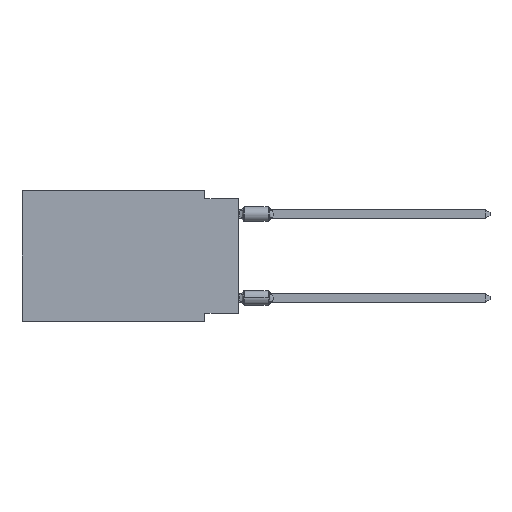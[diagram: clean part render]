
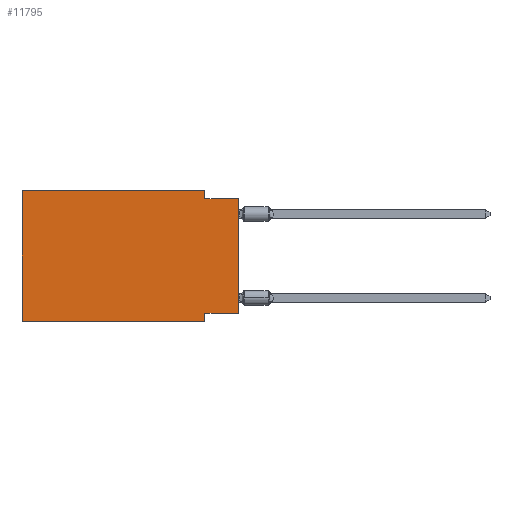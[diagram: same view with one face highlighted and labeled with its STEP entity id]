
A CAD part, left-side view. The second image highlights one B-rep face of the part: STEP entity #11795.
In plain terms, the highlighted planar face has unit normal (-1, 0, 0).
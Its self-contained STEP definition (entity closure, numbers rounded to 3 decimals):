
#19 = CARTESIAN_POINT ( 'NONE',  ( 0., 16.383, -9.906 ) ) ;
#109 = VECTOR ( 'NONE', #7532, 1000. ) ;
#499 = CARTESIAN_POINT ( 'NONE',  ( 0., 16.383, 0. ) ) ;
#580 = LINE ( 'NONE', #8457, #109 ) ;
#931 = EDGE_CURVE ( 'NONE', #2852, #11022, #6724, .T. ) ;
#1027 = DIRECTION ( 'NONE',  ( 0., -1., 0. ) ) ;
#1090 = LINE ( 'NONE', #4879, #1158 ) ;
#1113 = ORIENTED_EDGE ( 'NONE', *, *, #6436, .F. ) ;
#1158 = VECTOR ( 'NONE', #1027, 1000. ) ;
#1318 = ORIENTED_EDGE ( 'NONE', *, *, #931, .F. ) ;
#1481 = FACE_OUTER_BOUND ( 'NONE', #1704, .T. ) ;
#1704 = EDGE_LOOP ( 'NONE', ( #9704, #12590, #1318, #1113, #11437, #2610, #9833, #10017 ) ) ;
#1799 = DIRECTION ( 'NONE',  ( 0., 0., 1. ) ) ;
#1854 = LINE ( 'NONE', #12952, #9113 ) ;
#1952 = EDGE_CURVE ( 'NONE', #9389, #4710, #11287, .T. ) ;
#2149 = AXIS2_PLACEMENT_3D ( 'NONE', #499, #3488, #4475 ) ;
#2191 = LINE ( 'NONE', #7188, #9335 ) ;
#2273 = DIRECTION ( 'NONE',  ( 0., 0., 1. ) ) ;
#2501 = CARTESIAN_POINT ( 'NONE',  ( 0., 2.54, 0. ) ) ;
#2610 = ORIENTED_EDGE ( 'NONE', *, *, #7211, .T. ) ;
#2852 = VERTEX_POINT ( 'NONE', #6192 ) ;
#3065 = CARTESIAN_POINT ( 'NONE',  ( 0., 2.54, -0.635 ) ) ;
#3488 = DIRECTION ( 'NONE',  ( 1., 0., 0. ) ) ;
#3612 = CARTESIAN_POINT ( 'NONE',  ( 0., 16.383, 0. ) ) ;
#3860 = LINE ( 'NONE', #19, #9767 ) ;
#3903 = CARTESIAN_POINT ( 'NONE',  ( 0., 0., -0.635 ) ) ;
#4048 = EDGE_CURVE ( 'NONE', #9389, #7938, #2191, .T. ) ;
#4283 = EDGE_CURVE ( 'NONE', #8426, #10007, #1854, .T. ) ;
#4418 = DIRECTION ( 'NONE',  ( 0., 0., -1. ) ) ;
#4475 = DIRECTION ( 'NONE',  ( 0., 0., -1. ) ) ;
#4531 = CARTESIAN_POINT ( 'NONE',  ( 0., 0., -9.271 ) ) ;
#4710 = VERTEX_POINT ( 'NONE', #3903 ) ;
#4879 = CARTESIAN_POINT ( 'NONE',  ( 0., 16.383, 0. ) ) ;
#5300 = CARTESIAN_POINT ( 'NONE',  ( 0., 0., 0. ) ) ;
#5472 = PLANE ( 'NONE',  #2149 ) ;
#5849 = DIRECTION ( 'NONE',  ( 0., -1., 0. ) ) ;
#6192 = CARTESIAN_POINT ( 'NONE',  ( 0., 2.54, 0. ) ) ;
#6324 = VECTOR ( 'NONE', #6531, 1000. ) ;
#6436 = EDGE_CURVE ( 'NONE', #10007, #2852, #1090, .T. ) ;
#6531 = DIRECTION ( 'NONE',  ( 0., 0., -1. ) ) ;
#6724 = LINE ( 'NONE', #2501, #6324 ) ;
#6807 = CARTESIAN_POINT ( 'NONE',  ( 0., 2.54, -9.906 ) ) ;
#7188 = CARTESIAN_POINT ( 'NONE',  ( 0., 0., -9.271 ) ) ;
#7211 = EDGE_CURVE ( 'NONE', #8426, #9305, #3860, .T. ) ;
#7530 = LINE ( 'NONE', #10871, #7675 ) ;
#7532 = DIRECTION ( 'NONE',  ( 0., -1., 0. ) ) ;
#7675 = VECTOR ( 'NONE', #4418, 1000. ) ;
#7926 = EDGE_CURVE ( 'NONE', #7938, #9305, #7530, .T. ) ;
#7938 = VERTEX_POINT ( 'NONE', #11522 ) ;
#8426 = VERTEX_POINT ( 'NONE', #10123 ) ;
#8457 = CARTESIAN_POINT ( 'NONE',  ( 0., 0., -0.635 ) ) ;
#9113 = VECTOR ( 'NONE', #1799, 1000. ) ;
#9169 = EDGE_CURVE ( 'NONE', #11022, #4710, #580, .T. ) ;
#9289 = VECTOR ( 'NONE', #2273, 1000. ) ;
#9305 = VERTEX_POINT ( 'NONE', #6807 ) ;
#9335 = VECTOR ( 'NONE', #11190, 1000. ) ;
#9389 = VERTEX_POINT ( 'NONE', #4531 ) ;
#9704 = ORIENTED_EDGE ( 'NONE', *, *, #1952, .T. ) ;
#9767 = VECTOR ( 'NONE', #5849, 1000. ) ;
#9833 = ORIENTED_EDGE ( 'NONE', *, *, #7926, .F. ) ;
#10007 = VERTEX_POINT ( 'NONE', #3612 ) ;
#10017 = ORIENTED_EDGE ( 'NONE', *, *, #4048, .F. ) ;
#10123 = CARTESIAN_POINT ( 'NONE',  ( 0., 16.383, -9.906 ) ) ;
#10871 = CARTESIAN_POINT ( 'NONE',  ( 0., 2.54, -9.906 ) ) ;
#11022 = VERTEX_POINT ( 'NONE', #3065 ) ;
#11190 = DIRECTION ( 'NONE',  ( 0., 1., 0. ) ) ;
#11287 = LINE ( 'NONE', #5300, #9289 ) ;
#11437 = ORIENTED_EDGE ( 'NONE', *, *, #4283, .F. ) ;
#11522 = CARTESIAN_POINT ( 'NONE',  ( 0., 2.54, -9.271 ) ) ;
#11795 = ADVANCED_FACE ( 'NONE', ( #1481 ), #5472, .F. ) ;
#12590 = ORIENTED_EDGE ( 'NONE', *, *, #9169, .F. ) ;
#12952 = CARTESIAN_POINT ( 'NONE',  ( 0., 16.383, 0. ) ) ;
